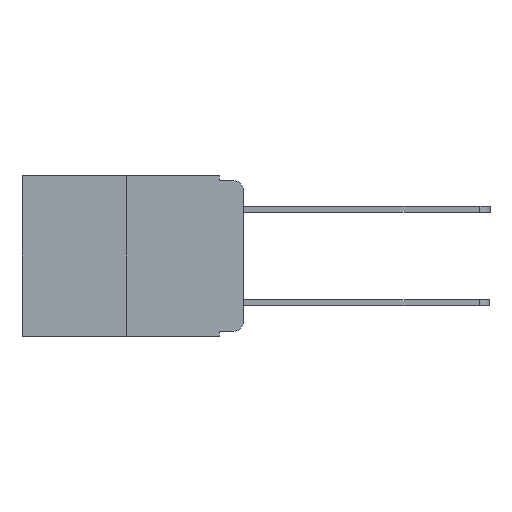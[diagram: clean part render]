
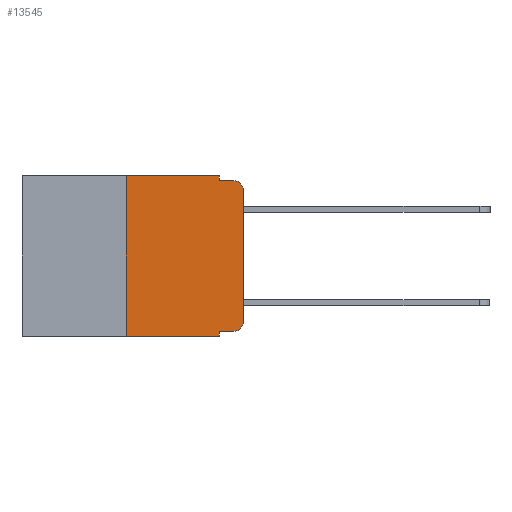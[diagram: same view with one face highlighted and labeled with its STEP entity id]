
A CAD part, left-side view. The second image highlights one B-rep face of the part: STEP entity #13545.
In plain terms, the highlighted planar face has unit normal (-1, 0, 0).
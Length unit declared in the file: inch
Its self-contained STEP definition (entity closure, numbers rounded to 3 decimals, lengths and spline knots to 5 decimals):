
#1020 = CARTESIAN_POINT ( 'NONE',  ( 0., 0.051, 0. ) ) ;
#1175 = CARTESIAN_POINT ( 'NONE',  ( 0., 0.02, -0.313 ) ) ;
#1489 = CARTESIAN_POINT ( 'NONE',  ( 0., 0.051, -0.333 ) ) ;
#1641 = DIRECTION ( 'NONE',  ( 0., -1., 0. ) ) ;
#2314 = EDGE_CURVE ( 'NONE', #10586, #8978, #4274, .T. ) ;
#2333 = ORIENTED_EDGE ( 'NONE', *, *, #13769, .F. ) ;
#2884 = DIRECTION ( 'NONE',  ( 0., 0., -1. ) ) ;
#2939 = DIRECTION ( 'NONE',  ( 0., 0., 1. ) ) ;
#3070 = AXIS2_PLACEMENT_3D ( 'NONE', #1175, #12735, #2884 ) ;
#3150 = LINE ( 'NONE', #4449, #11359 ) ;
#3210 = DIRECTION ( 'NONE',  ( 0., 0., 1. ) ) ;
#3260 = DIRECTION ( 'NONE',  ( 0., -1., 0. ) ) ;
#3525 = ORIENTED_EDGE ( 'NONE', *, *, #19996, .F. ) ;
#3755 = AXIS2_PLACEMENT_3D ( 'NONE', #17100, #7273, #18713 ) ;
#3923 = VERTEX_POINT ( 'NONE', #5961 ) ;
#3939 = VERTEX_POINT ( 'NONE', #4384 ) ;
#4274 = LINE ( 'NONE', #11111, #16845 ) ;
#4384 = CARTESIAN_POINT ( 'NONE',  ( 0., 0.02, -0.333 ) ) ;
#4449 = CARTESIAN_POINT ( 'NONE',  ( 0., 0.051, -0.01 ) ) ;
#5130 = VECTOR ( 'NONE', #15515, 39.37008 ) ;
#5550 = ORIENTED_EDGE ( 'NONE', *, *, #15944, .F. ) ;
#5915 = EDGE_CURVE ( 'NONE', #6144, #18335, #18191, .T. ) ;
#5961 = CARTESIAN_POINT ( 'NONE',  ( 0., 0.02, -0.01 ) ) ;
#6042 = DIRECTION ( 'NONE',  ( 0., 0., -1. ) ) ;
#6103 = DIRECTION ( 'NONE',  ( 0., -1., 0. ) ) ;
#6144 = VERTEX_POINT ( 'NONE', #12855 ) ;
#6556 = VECTOR ( 'NONE', #20831, 39.37008 ) ;
#6955 = ORIENTED_EDGE ( 'NONE', *, *, #5915, .T. ) ;
#7237 = PLANE ( 'NONE',  #19791 ) ;
#7273 = DIRECTION ( 'NONE',  ( -1., 0., 0. ) ) ;
#7323 = VERTEX_POINT ( 'NONE', #9647 ) ;
#8492 = LINE ( 'NONE', #15985, #20965 ) ;
#8503 = LINE ( 'NONE', #13184, #12362 ) ;
#8716 = LINE ( 'NONE', #1020, #12568 ) ;
#8829 = VERTEX_POINT ( 'NONE', #10123 ) ;
#8910 = DIRECTION ( 'NONE',  ( 0., 0., -1. ) ) ;
#8978 = VERTEX_POINT ( 'NONE', #13743 ) ;
#9140 = CIRCLE ( 'NONE', #3070, 0.02 ) ;
#9167 = EDGE_LOOP ( 'NONE', ( #13491, #16898, #11679, #16617, #3525, #5550, #6955, #2333, #14665, #11408 ) ) ;
#9184 = VECTOR ( 'NONE', #3260, 39.37008 ) ;
#9647 = CARTESIAN_POINT ( 'NONE',  ( 0., 0.051, -0.333 ) ) ;
#9692 = LINE ( 'NONE', #1489, #9184 ) ;
#10123 = CARTESIAN_POINT ( 'NONE',  ( 0., 0.051, -0.01 ) ) ;
#10438 = EDGE_CURVE ( 'NONE', #3939, #10586, #9140, .T. ) ;
#10586 = VERTEX_POINT ( 'NONE', #17925 ) ;
#11111 = CARTESIAN_POINT ( 'NONE',  ( 0., 0., 0. ) ) ;
#11359 = VECTOR ( 'NONE', #6103, 39.37008 ) ;
#11376 = VERTEX_POINT ( 'NONE', #16764 ) ;
#11408 = ORIENTED_EDGE ( 'NONE', *, *, #10438, .T. ) ;
#11679 = ORIENTED_EDGE ( 'NONE', *, *, #19189, .F. ) ;
#12362 = VECTOR ( 'NONE', #1641, 39.37008 ) ;
#12568 = VECTOR ( 'NONE', #6042, 39.37008 ) ;
#12653 = EDGE_CURVE ( 'NONE', #7323, #3939, #9692, .T. ) ;
#12735 = DIRECTION ( 'NONE',  ( -1., 0., 0. ) ) ;
#12855 = CARTESIAN_POINT ( 'NONE',  ( 0., 0.25, -0.343 ) ) ;
#13184 = CARTESIAN_POINT ( 'NONE',  ( 0., 0.473, 0. ) ) ;
#13491 = ORIENTED_EDGE ( 'NONE', *, *, #2314, .T. ) ;
#13545 = ADVANCED_FACE ( 'NONE', ( #18841 ), #7237, .F. ) ;
#13743 = CARTESIAN_POINT ( 'NONE',  ( 0., 0., -0.03 ) ) ;
#13769 = EDGE_CURVE ( 'NONE', #7323, #18335, #14280, .T. ) ;
#14280 = LINE ( 'NONE', #19231, #6556 ) ;
#14665 = ORIENTED_EDGE ( 'NONE', *, *, #12653, .T. ) ;
#15431 = CARTESIAN_POINT ( 'NONE',  ( 0., 0.473, 0. ) ) ;
#15515 = DIRECTION ( 'NONE',  ( 0., -1., 0. ) ) ;
#15944 = EDGE_CURVE ( 'NONE', #6144, #11376, #8492, .T. ) ;
#15985 = CARTESIAN_POINT ( 'NONE',  ( 0., 0.25, 0. ) ) ;
#16617 = ORIENTED_EDGE ( 'NONE', *, *, #17027, .F. ) ;
#16764 = CARTESIAN_POINT ( 'NONE',  ( 0., 0.25, 0. ) ) ;
#16845 = VECTOR ( 'NONE', #2939, 39.37008 ) ;
#16898 = ORIENTED_EDGE ( 'NONE', *, *, #20246, .T. ) ;
#17027 = EDGE_CURVE ( 'NONE', #21238, #8829, #8716, .T. ) ;
#17100 = CARTESIAN_POINT ( 'NONE',  ( 0., 0.02, -0.03 ) ) ;
#17151 = CARTESIAN_POINT ( 'NONE',  ( 0., 0.473, -0.343 ) ) ;
#17925 = CARTESIAN_POINT ( 'NONE',  ( 0., 0., -0.313 ) ) ;
#18191 = LINE ( 'NONE', #17151, #5130 ) ;
#18335 = VERTEX_POINT ( 'NONE', #20106 ) ;
#18681 = DIRECTION ( 'NONE',  ( 1., 0., 0. ) ) ;
#18713 = DIRECTION ( 'NONE',  ( 0., 0., -1. ) ) ;
#18841 = FACE_OUTER_BOUND ( 'NONE', #9167, .T. ) ;
#19189 = EDGE_CURVE ( 'NONE', #8829, #3923, #3150, .T. ) ;
#19231 = CARTESIAN_POINT ( 'NONE',  ( 0., 0.051, 0. ) ) ;
#19789 = CARTESIAN_POINT ( 'NONE',  ( 0., 0.051, 0. ) ) ;
#19791 = AXIS2_PLACEMENT_3D ( 'NONE', #15431, #18681, #8910 ) ;
#19996 = EDGE_CURVE ( 'NONE', #11376, #21238, #8503, .T. ) ;
#20106 = CARTESIAN_POINT ( 'NONE',  ( 0., 0.051, -0.343 ) ) ;
#20246 = EDGE_CURVE ( 'NONE', #8978, #3923, #20721, .T. ) ;
#20721 = CIRCLE ( 'NONE', #3755, 0.02 ) ;
#20831 = DIRECTION ( 'NONE',  ( 0., 0., -1. ) ) ;
#20965 = VECTOR ( 'NONE', #3210, 39.37008 ) ;
#21238 = VERTEX_POINT ( 'NONE', #19789 ) ;
